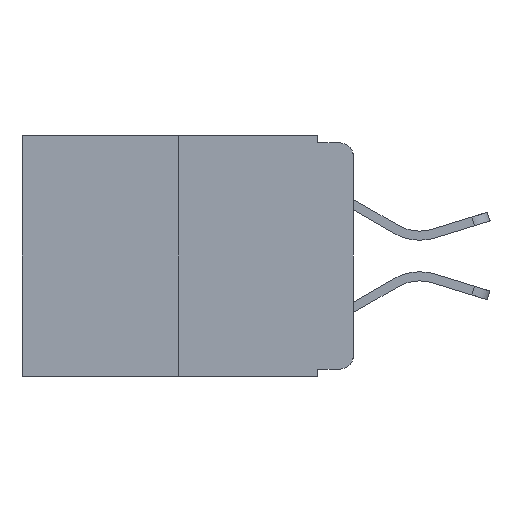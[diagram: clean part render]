
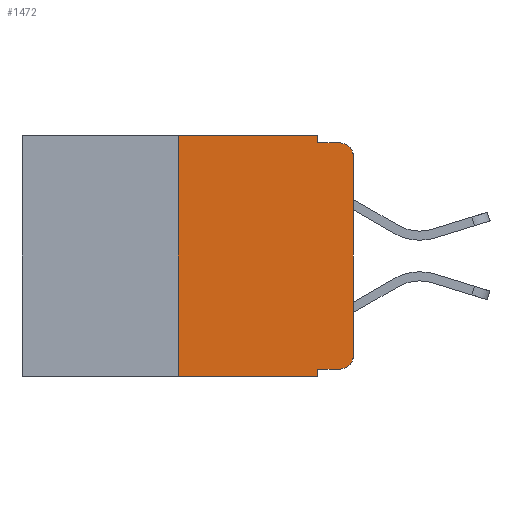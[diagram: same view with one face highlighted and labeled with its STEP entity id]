
A CAD part, left-side view. The second image highlights one B-rep face of the part: STEP entity #1472.
In plain terms, the highlighted planar face has unit normal (-1, 0, 0).
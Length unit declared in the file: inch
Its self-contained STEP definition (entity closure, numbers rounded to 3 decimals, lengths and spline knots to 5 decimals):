
#170 = CARTESIAN_POINT ( 'NONE',  ( 0., 0.473, -0.343 ) ) ;
#398 = CARTESIAN_POINT ( 'NONE',  ( 0., 0.051, -0.333 ) ) ;
#444 = VECTOR ( 'NONE', #1274, 39.37008 ) ;
#703 = VERTEX_POINT ( 'NONE', #12379 ) ;
#819 = CARTESIAN_POINT ( 'NONE',  ( 0., 0.051, -0.333 ) ) ;
#946 = CARTESIAN_POINT ( 'NONE',  ( 0., 0.25, 0. ) ) ;
#1274 = DIRECTION ( 'NONE',  ( 0., 0., -1. ) ) ;
#1314 = CARTESIAN_POINT ( 'NONE',  ( 0., 0.051, 0. ) ) ;
#1472 = ADVANCED_FACE ( 'NONE', ( #8795 ), #6736, .F. ) ;
#1479 = AXIS2_PLACEMENT_3D ( 'NONE', #3716, #7775, #9883 ) ;
#1789 = DIRECTION ( 'NONE',  ( 0., -1., 0. ) ) ;
#1816 = EDGE_CURVE ( 'NONE', #7812, #9264, #6624, .T. ) ;
#1919 = VECTOR ( 'NONE', #1943, 39.37008 ) ;
#1940 = ORIENTED_EDGE ( 'NONE', *, *, #6883, .F. ) ;
#1943 = DIRECTION ( 'NONE',  ( 0., -1., 0. ) ) ;
#1974 = ORIENTED_EDGE ( 'NONE', *, *, #11637, .F. ) ;
#2125 = CARTESIAN_POINT ( 'NONE',  ( 0., 0.02, -0.333 ) ) ;
#2369 = EDGE_LOOP ( 'NONE', ( #8528, #8264, #6630, #7979, #1974, #6215, #6466, #1940, #5625, #11303 ) ) ;
#2746 = AXIS2_PLACEMENT_3D ( 'NONE', #5992, #6387, #11327 ) ;
#3046 = DIRECTION ( 'NONE',  ( 0., -1., 0. ) ) ;
#3181 = AXIS2_PLACEMENT_3D ( 'NONE', #9311, #9242, #9192 ) ;
#3304 = VERTEX_POINT ( 'NONE', #8185 ) ;
#3655 = CARTESIAN_POINT ( 'NONE',  ( 0., 0.051, -0.343 ) ) ;
#3657 = CARTESIAN_POINT ( 'NONE',  ( 0., 0.051, 0. ) ) ;
#3688 = VECTOR ( 'NONE', #5355, 39.37008 ) ;
#3716 = CARTESIAN_POINT ( 'NONE',  ( 0., 0.02, -0.313 ) ) ;
#3795 = VECTOR ( 'NONE', #1789, 39.37008 ) ;
#3815 = VERTEX_POINT ( 'NONE', #11427 ) ;
#3906 = CARTESIAN_POINT ( 'NONE',  ( 0., 0.473, 0. ) ) ;
#3976 = EDGE_CURVE ( 'NONE', #3304, #5866, #6708, .T. ) ;
#4654 = LINE ( 'NONE', #9939, #9629 ) ;
#5013 = VERTEX_POINT ( 'NONE', #3655 ) ;
#5102 = EDGE_CURVE ( 'NONE', #5675, #703, #8047, .T. ) ;
#5323 = EDGE_CURVE ( 'NONE', #10331, #5675, #4654, .T. ) ;
#5355 = DIRECTION ( 'NONE',  ( 0., 0., 1. ) ) ;
#5386 = CARTESIAN_POINT ( 'NONE',  ( 0., 0.051, -0.01 ) ) ;
#5590 = EDGE_CURVE ( 'NONE', #3304, #5013, #6542, .T. ) ;
#5625 = ORIENTED_EDGE ( 'NONE', *, *, #9870, .T. ) ;
#5675 = VERTEX_POINT ( 'NONE', #5386 ) ;
#5866 = VERTEX_POINT ( 'NONE', #10540 ) ;
#5992 = CARTESIAN_POINT ( 'NONE',  ( 0., 0.473, 0. ) ) ;
#6162 = EDGE_CURVE ( 'NONE', #3815, #703, #10722, .T. ) ;
#6215 = ORIENTED_EDGE ( 'NONE', *, *, #3976, .F. ) ;
#6247 = VECTOR ( 'NONE', #3046, 39.37008 ) ;
#6343 = CARTESIAN_POINT ( 'NONE',  ( 0., 0.051, -0.01 ) ) ;
#6362 = LINE ( 'NONE', #11700, #3688 ) ;
#6387 = DIRECTION ( 'NONE',  ( 1., 0., 0. ) ) ;
#6466 = ORIENTED_EDGE ( 'NONE', *, *, #5590, .T. ) ;
#6542 = LINE ( 'NONE', #170, #6247 ) ;
#6624 = CIRCLE ( 'NONE', #1479, 0.02 ) ;
#6630 = ORIENTED_EDGE ( 'NONE', *, *, #5102, .F. ) ;
#6708 = LINE ( 'NONE', #946, #10897 ) ;
#6736 = PLANE ( 'NONE',  #2746 ) ;
#6883 = EDGE_CURVE ( 'NONE', #9613, #5013, #8551, .T. ) ;
#7775 = DIRECTION ( 'NONE',  ( -1., 0., 0. ) ) ;
#7812 = VERTEX_POINT ( 'NONE', #2125 ) ;
#7858 = EDGE_CURVE ( 'NONE', #9264, #3815, #6362, .T. ) ;
#7979 = ORIENTED_EDGE ( 'NONE', *, *, #5323, .F. ) ;
#8047 = LINE ( 'NONE', #6343, #8332 ) ;
#8185 = CARTESIAN_POINT ( 'NONE',  ( 0., 0.25, -0.343 ) ) ;
#8264 = ORIENTED_EDGE ( 'NONE', *, *, #6162, .T. ) ;
#8268 = DIRECTION ( 'NONE',  ( 0., -1., 0. ) ) ;
#8332 = VECTOR ( 'NONE', #8268, 39.37008 ) ;
#8528 = ORIENTED_EDGE ( 'NONE', *, *, #7858, .T. ) ;
#8551 = LINE ( 'NONE', #1314, #444 ) ;
#8626 = LINE ( 'NONE', #3906, #3795 ) ;
#8795 = FACE_OUTER_BOUND ( 'NONE', #2369, .T. ) ;
#9010 = CARTESIAN_POINT ( 'NONE',  ( 0., 0., -0.313 ) ) ;
#9192 = DIRECTION ( 'NONE',  ( 0., 0., -1. ) ) ;
#9242 = DIRECTION ( 'NONE',  ( -1., 0., 0. ) ) ;
#9264 = VERTEX_POINT ( 'NONE', #9010 ) ;
#9311 = CARTESIAN_POINT ( 'NONE',  ( 0., 0.02, -0.03 ) ) ;
#9613 = VERTEX_POINT ( 'NONE', #398 ) ;
#9629 = VECTOR ( 'NONE', #9917, 39.37008 ) ;
#9870 = EDGE_CURVE ( 'NONE', #9613, #7812, #12277, .T. ) ;
#9883 = DIRECTION ( 'NONE',  ( 0., 0., -1. ) ) ;
#9917 = DIRECTION ( 'NONE',  ( 0., 0., -1. ) ) ;
#9939 = CARTESIAN_POINT ( 'NONE',  ( 0., 0.051, 0. ) ) ;
#10331 = VERTEX_POINT ( 'NONE', #3657 ) ;
#10540 = CARTESIAN_POINT ( 'NONE',  ( 0., 0.25, 0. ) ) ;
#10722 = CIRCLE ( 'NONE', #3181, 0.02 ) ;
#10897 = VECTOR ( 'NONE', #12187, 39.37008 ) ;
#11303 = ORIENTED_EDGE ( 'NONE', *, *, #1816, .T. ) ;
#11327 = DIRECTION ( 'NONE',  ( 0., 0., -1. ) ) ;
#11427 = CARTESIAN_POINT ( 'NONE',  ( 0., 0., -0.03 ) ) ;
#11637 = EDGE_CURVE ( 'NONE', #5866, #10331, #8626, .T. ) ;
#11700 = CARTESIAN_POINT ( 'NONE',  ( 0., 0., 0. ) ) ;
#12187 = DIRECTION ( 'NONE',  ( 0., 0., 1. ) ) ;
#12277 = LINE ( 'NONE', #819, #1919 ) ;
#12379 = CARTESIAN_POINT ( 'NONE',  ( 0., 0.02, -0.01 ) ) ;
